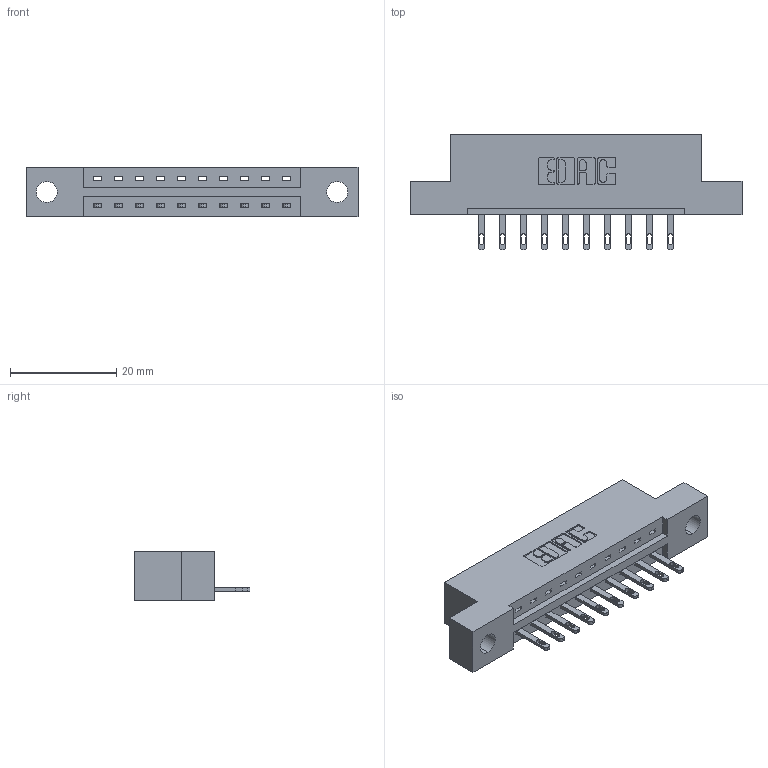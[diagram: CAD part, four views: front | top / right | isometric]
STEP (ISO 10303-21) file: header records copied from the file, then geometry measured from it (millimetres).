
FILE_DESCRIPTION (( 'STEP AP203' ), '1' );
FILE_NAME ('337-010-500-104.STEP', '2019-09-27T20:48:18', ( '' ), ( '' ), 'SwSTEP 2.0', 'SolidWorks 2016', '' );
FILE_SCHEMA (( 'CONFIG_CONTROL_DESIGN' ));
Length unit declared in the file: inch
Products named in the file (3): 337 Part_Flush Mounting Lugs - 0.156 Dia-TH; 337-010-500-104; 345-292-001_345-293-100
Assembly tree (11 placements, depth 2):
  337-010-500-104
    337 Part_Flush Mounting Lugs - 0.156 Dia-TH
    345-292-001_345-293-100  x10
Bounding box: 62.64 x 21.85 x 9.4 mm (x, y, z)
Volume: 6027.9 mm3; surface area: 5870 mm2
Topology: 11 solids, 11 shells, 694 faces, 2111 edges, 1406 vertices
Faces by surface type: plane 470, cylinder 224
Entity records: 11505 total; most frequent: CARTESIAN_POINT 2008, ORIENTED_EDGE 1954, DIRECTION 1757, EDGE_CURVE 977, LINE 845, VECTOR 845, VERTEX_POINT 650, AXIS2_PLACEMENT_3D 456
